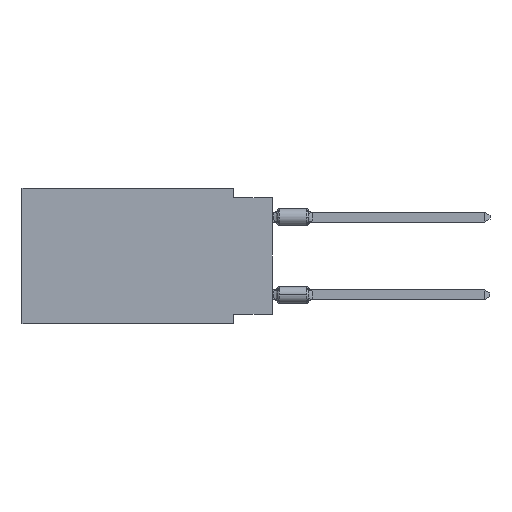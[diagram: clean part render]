
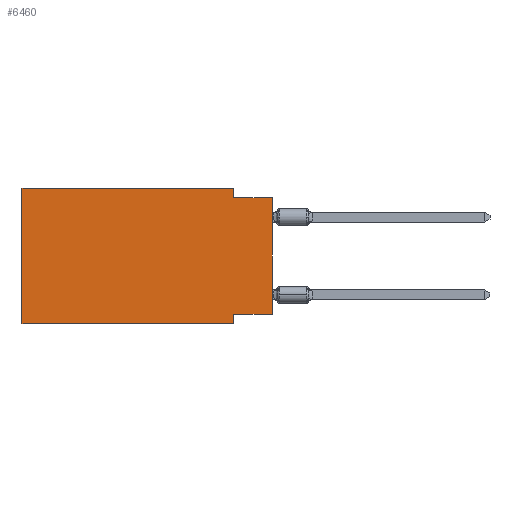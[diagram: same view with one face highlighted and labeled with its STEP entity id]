
A CAD part, left-side view. The second image highlights one B-rep face of the part: STEP entity #6460.
In plain terms, the highlighted planar face has unit normal (-1, 0, 0).
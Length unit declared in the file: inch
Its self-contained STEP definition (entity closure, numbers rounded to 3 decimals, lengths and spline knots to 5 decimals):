
#91 = VERTEX_POINT ( 'NONE', #2884 ) ;
#197 = CARTESIAN_POINT ( 'NONE',  ( 0., 0.645, 0. ) ) ;
#395 = VERTEX_POINT ( 'NONE', #5063 ) ;
#679 = ORIENTED_EDGE ( 'NONE', *, *, #1974, .F. ) ;
#1008 = VERTEX_POINT ( 'NONE', #7926 ) ;
#1040 = CARTESIAN_POINT ( 'NONE',  ( 0., 0.645, 0. ) ) ;
#1136 = ORIENTED_EDGE ( 'NONE', *, *, #4383, .F. ) ;
#1211 = FACE_OUTER_BOUND ( 'NONE', #11921, .T. ) ;
#1267 = ORIENTED_EDGE ( 'NONE', *, *, #10711, .F. ) ;
#1379 = DIRECTION ( 'NONE',  ( 1., 0., 0. ) ) ;
#1561 = ORIENTED_EDGE ( 'NONE', *, *, #4725, .T. ) ;
#1729 = ORIENTED_EDGE ( 'NONE', *, *, #6033, .F. ) ;
#1974 = EDGE_CURVE ( 'NONE', #11878, #7509, #2015, .T. ) ;
#1988 = EDGE_CURVE ( 'NONE', #395, #91, #3360, .T. ) ;
#2015 = LINE ( 'NONE', #7186, #5535 ) ;
#2569 = PLANE ( 'NONE',  #9409 ) ;
#2884 = CARTESIAN_POINT ( 'NONE',  ( 0., 0.645, 0. ) ) ;
#3021 = CARTESIAN_POINT ( 'NONE',  ( 0., 0., 0. ) ) ;
#3232 = EDGE_CURVE ( 'NONE', #11878, #1008, #5646, .T. ) ;
#3360 = LINE ( 'NONE', #13820, #3378 ) ;
#3378 = VECTOR ( 'NONE', #16546, 39.37008 ) ;
#3624 = CARTESIAN_POINT ( 'NONE',  ( 0., 0.645, -0.35 ) ) ;
#3897 = DIRECTION ( 'NONE',  ( 0., 0., -1. ) ) ;
#4240 = VECTOR ( 'NONE', #13983, 39.37008 ) ;
#4302 = CARTESIAN_POINT ( 'NONE',  ( 0., 0.1, -0.325 ) ) ;
#4383 = EDGE_CURVE ( 'NONE', #91, #7878, #7482, .T. ) ;
#4661 = ORIENTED_EDGE ( 'NONE', *, *, #3232, .T. ) ;
#4713 = CARTESIAN_POINT ( 'NONE',  ( 0., 0.1, 0. ) ) ;
#4725 = EDGE_CURVE ( 'NONE', #395, #6755, #16793, .T. ) ;
#5063 = CARTESIAN_POINT ( 'NONE',  ( 0., 0.645, -0.35 ) ) ;
#5427 = LINE ( 'NONE', #15562, #11113 ) ;
#5535 = VECTOR ( 'NONE', #12361, 39.37008 ) ;
#5646 = LINE ( 'NONE', #3021, #12316 ) ;
#6033 = EDGE_CURVE ( 'NONE', #7878, #16703, #8795, .T. ) ;
#6045 = VECTOR ( 'NONE', #12973, 39.37008 ) ;
#6460 = ADVANCED_FACE ( 'NONE', ( #1211 ), #2569, .F. ) ;
#6755 = VERTEX_POINT ( 'NONE', #8672 ) ;
#7186 = CARTESIAN_POINT ( 'NONE',  ( 0., 0., -0.325 ) ) ;
#7482 = LINE ( 'NONE', #1040, #9687 ) ;
#7509 = VERTEX_POINT ( 'NONE', #4302 ) ;
#7529 = DIRECTION ( 'NONE',  ( 0., -1., 0. ) ) ;
#7586 = CARTESIAN_POINT ( 'NONE',  ( 0., 0.1, -0.025 ) ) ;
#7878 = VERTEX_POINT ( 'NONE', #14607 ) ;
#7926 = CARTESIAN_POINT ( 'NONE',  ( 0., 0., -0.025 ) ) ;
#8672 = CARTESIAN_POINT ( 'NONE',  ( 0., 0.1, -0.35 ) ) ;
#8795 = LINE ( 'NONE', #4713, #4240 ) ;
#9287 = CARTESIAN_POINT ( 'NONE',  ( 0., 0., -0.325 ) ) ;
#9409 = AXIS2_PLACEMENT_3D ( 'NONE', #197, #1379, #10374 ) ;
#9679 = VECTOR ( 'NONE', #7529, 39.37008 ) ;
#9687 = VECTOR ( 'NONE', #12754, 39.37008 ) ;
#10374 = DIRECTION ( 'NONE',  ( 0., 0., -1. ) ) ;
#10447 = ORIENTED_EDGE ( 'NONE', *, *, #1988, .F. ) ;
#10711 = EDGE_CURVE ( 'NONE', #16703, #1008, #15534, .T. ) ;
#11113 = VECTOR ( 'NONE', #3897, 39.37008 ) ;
#11878 = VERTEX_POINT ( 'NONE', #9287 ) ;
#11921 = EDGE_LOOP ( 'NONE', ( #4661, #1267, #1729, #1136, #10447, #1561, #16294, #679 ) ) ;
#12316 = VECTOR ( 'NONE', #13560, 39.37008 ) ;
#12361 = DIRECTION ( 'NONE',  ( 0., 1., 0. ) ) ;
#12618 = CARTESIAN_POINT ( 'NONE',  ( 0., 0., -0.025 ) ) ;
#12754 = DIRECTION ( 'NONE',  ( 0., -1., 0. ) ) ;
#12973 = DIRECTION ( 'NONE',  ( 0., -1., 0. ) ) ;
#13560 = DIRECTION ( 'NONE',  ( 0., 0., 1. ) ) ;
#13820 = CARTESIAN_POINT ( 'NONE',  ( 0., 0.645, 0. ) ) ;
#13983 = DIRECTION ( 'NONE',  ( 0., 0., -1. ) ) ;
#14334 = EDGE_CURVE ( 'NONE', #7509, #6755, #5427, .T. ) ;
#14607 = CARTESIAN_POINT ( 'NONE',  ( 0., 0.1, 0. ) ) ;
#15534 = LINE ( 'NONE', #12618, #6045 ) ;
#15562 = CARTESIAN_POINT ( 'NONE',  ( 0., 0.1, -0.35 ) ) ;
#16294 = ORIENTED_EDGE ( 'NONE', *, *, #14334, .F. ) ;
#16546 = DIRECTION ( 'NONE',  ( 0., 0., 1. ) ) ;
#16703 = VERTEX_POINT ( 'NONE', #7586 ) ;
#16793 = LINE ( 'NONE', #3624, #9679 ) ;
